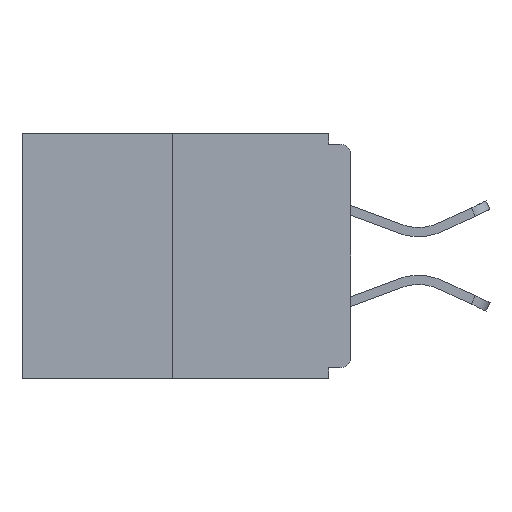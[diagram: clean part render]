
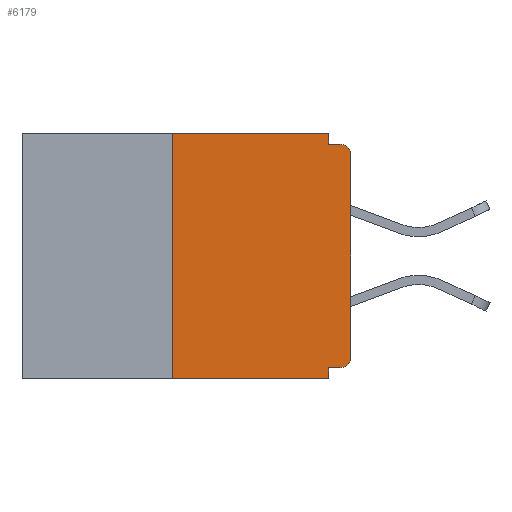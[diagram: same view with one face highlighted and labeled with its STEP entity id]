
A CAD part, left-side view. The second image highlights one B-rep face of the part: STEP entity #6179.
In plain terms, the highlighted planar face has unit normal (-1, 0, 0).
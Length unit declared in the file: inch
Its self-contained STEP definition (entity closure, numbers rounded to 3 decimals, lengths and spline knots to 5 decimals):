
#15 = CARTESIAN_POINT ( 'NONE',  ( 0., 0.015, -0.313 ) ) ;
#333 = DIRECTION ( 'NONE',  ( 0., 0., -1. ) ) ;
#597 = VERTEX_POINT ( 'NONE', #10854 ) ;
#1139 = CARTESIAN_POINT ( 'NONE',  ( 0., 0., -0.015 ) ) ;
#1315 = DIRECTION ( 'NONE',  ( 0., 0., 1. ) ) ;
#1393 = ORIENTED_EDGE ( 'NONE', *, *, #15376, .F. ) ;
#1577 = ORIENTED_EDGE ( 'NONE', *, *, #13887, .F. ) ;
#2232 = ORIENTED_EDGE ( 'NONE', *, *, #6409, .T. ) ;
#2328 = DIRECTION ( 'NONE',  ( 0., -1., 0. ) ) ;
#2338 = LINE ( 'NONE', #9472, #17141 ) ;
#2629 = CIRCLE ( 'NONE', #9040, 0.015 ) ;
#2793 = DIRECTION ( 'NONE',  ( 0., -1., 0. ) ) ;
#2834 = DIRECTION ( 'NONE',  ( 0., 0., -1. ) ) ;
#3137 = EDGE_CURVE ( 'NONE', #16726, #17376, #6424, .T. ) ;
#3198 = DIRECTION ( 'NONE',  ( 0., 0., -1. ) ) ;
#3591 = VECTOR ( 'NONE', #1315, 39.37008 ) ;
#3693 = EDGE_CURVE ( 'NONE', #17376, #17039, #10971, .T. ) ;
#3955 = CARTESIAN_POINT ( 'NONE',  ( 0., 0.46, -0.343 ) ) ;
#4075 = VERTEX_POINT ( 'NONE', #17555 ) ;
#4153 = CARTESIAN_POINT ( 'NONE',  ( 0., 0., 0. ) ) ;
#4253 = ORIENTED_EDGE ( 'NONE', *, *, #16607, .T. ) ;
#4662 = CARTESIAN_POINT ( 'NONE',  ( 0., 0., -0.313 ) ) ;
#4688 = FACE_OUTER_BOUND ( 'NONE', #12695, .T. ) ;
#4721 = CARTESIAN_POINT ( 'NONE',  ( 0., 0.031, -0.343 ) ) ;
#5090 = CARTESIAN_POINT ( 'NONE',  ( 0., 0.031, -0.343 ) ) ;
#5381 = EDGE_CURVE ( 'NONE', #597, #8972, #2338, .T. ) ;
#5397 = DIRECTION ( 'NONE',  ( 0., 0., -1. ) ) ;
#5485 = ORIENTED_EDGE ( 'NONE', *, *, #17788, .F. ) ;
#6179 = ADVANCED_FACE ( 'NONE', ( #4688 ), #13105, .F. ) ;
#6409 = EDGE_CURVE ( 'NONE', #10071, #15255, #14687, .T. ) ;
#6424 = LINE ( 'NONE', #10247, #3591 ) ;
#6729 = LINE ( 'NONE', #3955, #9959 ) ;
#6997 = CARTESIAN_POINT ( 'NONE',  ( 0., 0.031, 0. ) ) ;
#7456 = VECTOR ( 'NONE', #333, 39.37008 ) ;
#8110 = CARTESIAN_POINT ( 'NONE',  ( 0., 0.015, -0.03 ) ) ;
#8546 = CIRCLE ( 'NONE', #18026, 0.015 ) ;
#8710 = VECTOR ( 'NONE', #2793, 39.37008 ) ;
#8757 = LINE ( 'NONE', #4721, #7456 ) ;
#8972 = VERTEX_POINT ( 'NONE', #10859 ) ;
#9040 = AXIS2_PLACEMENT_3D ( 'NONE', #8110, #10920, #5397 ) ;
#9151 = CARTESIAN_POINT ( 'NONE',  ( 0., 0., -0.03 ) ) ;
#9472 = CARTESIAN_POINT ( 'NONE',  ( 0., 0., -0.328 ) ) ;
#9634 = CARTESIAN_POINT ( 'NONE',  ( 0., 0.46, 0. ) ) ;
#9785 = DIRECTION ( 'NONE',  ( 0., 0., 1. ) ) ;
#9791 = LINE ( 'NONE', #1139, #8710 ) ;
#9959 = VECTOR ( 'NONE', #2328, 39.37008 ) ;
#10071 = VERTEX_POINT ( 'NONE', #4662 ) ;
#10156 = CARTESIAN_POINT ( 'NONE',  ( 0., 0.031, 0. ) ) ;
#10247 = CARTESIAN_POINT ( 'NONE',  ( 0., 0.25, 0. ) ) ;
#10617 = EDGE_CURVE ( 'NONE', #16726, #17549, #6729, .T. ) ;
#10854 = CARTESIAN_POINT ( 'NONE',  ( 0., 0.015, -0.328 ) ) ;
#10859 = CARTESIAN_POINT ( 'NONE',  ( 0., 0.031, -0.328 ) ) ;
#10920 = DIRECTION ( 'NONE',  ( -1., 0., 0. ) ) ;
#10971 = LINE ( 'NONE', #9634, #14893 ) ;
#11017 = VECTOR ( 'NONE', #3198, 39.37008 ) ;
#11026 = DIRECTION ( 'NONE',  ( 0., 0., -1. ) ) ;
#11108 = ORIENTED_EDGE ( 'NONE', *, *, #5381, .F. ) ;
#11123 = AXIS2_PLACEMENT_3D ( 'NONE', #17935, #16555, #11026 ) ;
#12571 = DIRECTION ( 'NONE',  ( 0., -1., 0. ) ) ;
#12695 = EDGE_LOOP ( 'NONE', ( #17592, #13004, #18067, #1577, #11108, #14057, #2232, #4253, #1393, #5485 ) ) ;
#13004 = ORIENTED_EDGE ( 'NONE', *, *, #3137, .F. ) ;
#13105 = PLANE ( 'NONE',  #11123 ) ;
#13268 = EDGE_CURVE ( 'NONE', #597, #10071, #8546, .T. ) ;
#13887 = EDGE_CURVE ( 'NONE', #8972, #17549, #8757, .T. ) ;
#14057 = ORIENTED_EDGE ( 'NONE', *, *, #13268, .T. ) ;
#14379 = CARTESIAN_POINT ( 'NONE',  ( 0., 0.25, -0.343 ) ) ;
#14687 = LINE ( 'NONE', #4153, #15979 ) ;
#14696 = CARTESIAN_POINT ( 'NONE',  ( 0., 0.25, 0. ) ) ;
#14893 = VECTOR ( 'NONE', #12571, 39.37008 ) ;
#15255 = VERTEX_POINT ( 'NONE', #9151 ) ;
#15376 = EDGE_CURVE ( 'NONE', #16309, #4075, #9791, .T. ) ;
#15393 = DIRECTION ( 'NONE',  ( -1., 0., 0. ) ) ;
#15638 = CARTESIAN_POINT ( 'NONE',  ( 0., 0.031, -0.015 ) ) ;
#15979 = VECTOR ( 'NONE', #9785, 39.37008 ) ;
#16309 = VERTEX_POINT ( 'NONE', #15638 ) ;
#16555 = DIRECTION ( 'NONE',  ( 1., 0., 0. ) ) ;
#16607 = EDGE_CURVE ( 'NONE', #15255, #4075, #2629, .T. ) ;
#16726 = VERTEX_POINT ( 'NONE', #14379 ) ;
#17039 = VERTEX_POINT ( 'NONE', #6997 ) ;
#17141 = VECTOR ( 'NONE', #17722, 39.37008 ) ;
#17376 = VERTEX_POINT ( 'NONE', #14696 ) ;
#17549 = VERTEX_POINT ( 'NONE', #5090 ) ;
#17555 = CARTESIAN_POINT ( 'NONE',  ( 0., 0.015, -0.015 ) ) ;
#17592 = ORIENTED_EDGE ( 'NONE', *, *, #3693, .F. ) ;
#17722 = DIRECTION ( 'NONE',  ( 0., 1., 0. ) ) ;
#17788 = EDGE_CURVE ( 'NONE', #17039, #16309, #18028, .T. ) ;
#17935 = CARTESIAN_POINT ( 'NONE',  ( 0., 0.46, 0. ) ) ;
#18026 = AXIS2_PLACEMENT_3D ( 'NONE', #15, #15393, #2834 ) ;
#18028 = LINE ( 'NONE', #10156, #11017 ) ;
#18067 = ORIENTED_EDGE ( 'NONE', *, *, #10617, .T. ) ;
